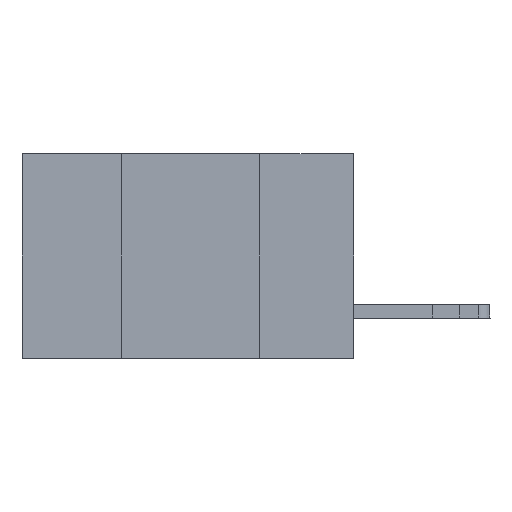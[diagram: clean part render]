
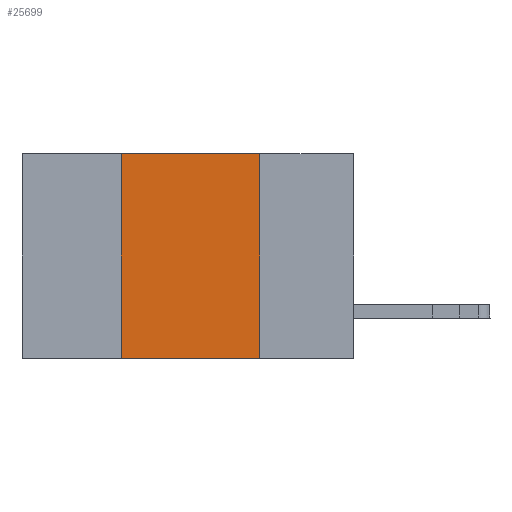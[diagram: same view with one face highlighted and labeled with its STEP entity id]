
A CAD part, left-side view. The second image highlights one B-rep face of the part: STEP entity #25699.
In plain terms, the highlighted planar face has unit normal (-1, 0, 0).
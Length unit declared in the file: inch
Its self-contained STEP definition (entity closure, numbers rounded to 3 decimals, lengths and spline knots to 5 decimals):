
#1677 = CARTESIAN_POINT ( 'NONE',  ( 0., 0.17, -0.37 ) ) ;
#1870 = LINE ( 'NONE', #28125, #7043 ) ;
#1896 = EDGE_CURVE ( 'NONE', #23996, #30379, #1870, .T. ) ;
#2559 = LINE ( 'NONE', #24095, #12951 ) ;
#6350 = CARTESIAN_POINT ( 'NONE',  ( 0., 0.6, 0. ) ) ;
#7043 = VECTOR ( 'NONE', #34170, 39.37008 ) ;
#11140 = ORIENTED_EDGE ( 'NONE', *, *, #20056, .F. ) ;
#11252 = CARTESIAN_POINT ( 'NONE',  ( 0., 0.17, 0. ) ) ;
#12951 = VECTOR ( 'NONE', #27123, 39.37008 ) ;
#13317 = VECTOR ( 'NONE', #29145, 39.37008 ) ;
#16500 = LINE ( 'NONE', #18212, #26362 ) ;
#17734 = AXIS2_PLACEMENT_3D ( 'NONE', #6350, #30461, #34225 ) ;
#18212 = CARTESIAN_POINT ( 'NONE',  ( 0., 0.6, -0.37 ) ) ;
#18913 = EDGE_LOOP ( 'NONE', ( #20525, #11140, #21452, #38912 ) ) ;
#19594 = VERTEX_POINT ( 'NONE', #11252 ) ;
#20056 = EDGE_CURVE ( 'NONE', #30379, #19594, #29334, .T. ) ;
#20525 = ORIENTED_EDGE ( 'NONE', *, *, #38271, .F. ) ;
#21452 = ORIENTED_EDGE ( 'NONE', *, *, #1896, .F. ) ;
#23996 = VERTEX_POINT ( 'NONE', #35146 ) ;
#24095 = CARTESIAN_POINT ( 'NONE',  ( 0., 0.17, 0. ) ) ;
#24226 = DIRECTION ( 'NONE',  ( 0., -1., 0. ) ) ;
#25560 = CARTESIAN_POINT ( 'NONE',  ( 0., 0.42, 0. ) ) ;
#25699 = ADVANCED_FACE ( 'NONE', ( #38105 ), #26668, .F. ) ;
#26362 = VECTOR ( 'NONE', #24226, 39.37008 ) ;
#26668 = PLANE ( 'NONE',  #17734 ) ;
#27123 = DIRECTION ( 'NONE',  ( 0., 0., -1. ) ) ;
#27467 = VERTEX_POINT ( 'NONE', #1677 ) ;
#28125 = CARTESIAN_POINT ( 'NONE',  ( 0., 0.42, 0. ) ) ;
#29145 = DIRECTION ( 'NONE',  ( 0., -1., 0. ) ) ;
#29334 = LINE ( 'NONE', #37567, #13317 ) ;
#30379 = VERTEX_POINT ( 'NONE', #25560 ) ;
#30461 = DIRECTION ( 'NONE',  ( 1., 0., 0. ) ) ;
#34170 = DIRECTION ( 'NONE',  ( 0., 0., 1. ) ) ;
#34225 = DIRECTION ( 'NONE',  ( 0., 0., -1. ) ) ;
#35122 = EDGE_CURVE ( 'NONE', #23996, #27467, #16500, .T. ) ;
#35146 = CARTESIAN_POINT ( 'NONE',  ( 0., 0.42, -0.37 ) ) ;
#37567 = CARTESIAN_POINT ( 'NONE',  ( 0., 0.6, 0. ) ) ;
#38105 = FACE_OUTER_BOUND ( 'NONE', #18913, .T. ) ;
#38271 = EDGE_CURVE ( 'NONE', #19594, #27467, #2559, .T. ) ;
#38912 = ORIENTED_EDGE ( 'NONE', *, *, #35122, .T. ) ;
